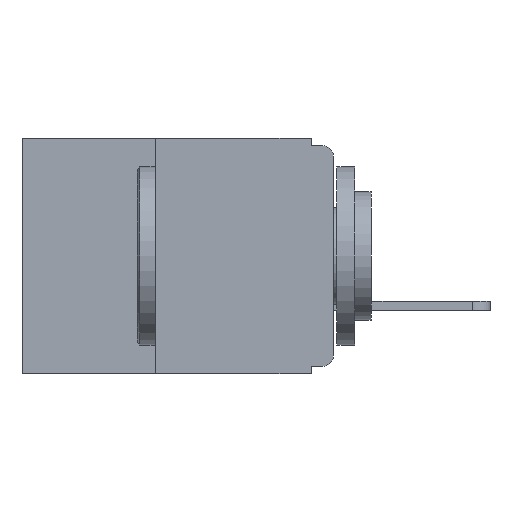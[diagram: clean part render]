
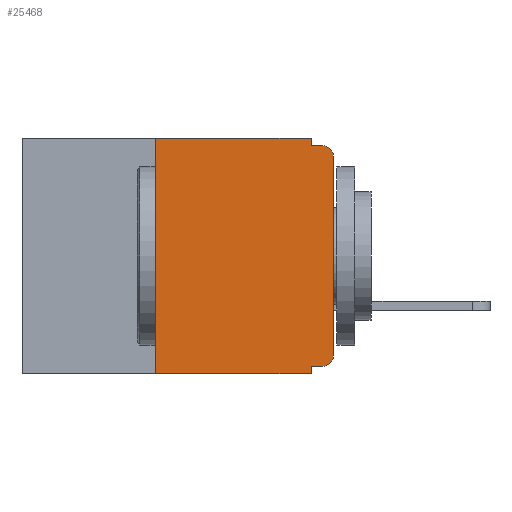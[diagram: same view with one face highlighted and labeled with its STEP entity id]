
A CAD part, left-side view. The second image highlights one B-rep face of the part: STEP entity #25468.
In plain terms, the highlighted planar face has unit normal (-1, 0, 0).
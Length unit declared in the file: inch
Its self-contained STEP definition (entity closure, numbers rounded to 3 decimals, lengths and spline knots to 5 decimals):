
#475 = CIRCLE ( 'NONE', #19467, 0.015 ) ;
#1059 = VERTEX_POINT ( 'NONE', #14954 ) ;
#1251 = DIRECTION ( 'NONE',  ( -1., 0., 0. ) ) ;
#1828 = LINE ( 'NONE', #4711, #18240 ) ;
#1950 = CARTESIAN_POINT ( 'NONE',  ( 0., 0.015, -0.32 ) ) ;
#2035 = AXIS2_PLACEMENT_3D ( 'NONE', #14182, #1251, #16287 ) ;
#2042 = CARTESIAN_POINT ( 'NONE',  ( 0., 0.437, 0. ) ) ;
#2110 = CARTESIAN_POINT ( 'NONE',  ( 0., 0., -0.01 ) ) ;
#2238 = CARTESIAN_POINT ( 'NONE',  ( 0., 0., 0. ) ) ;
#2360 = EDGE_CURVE ( 'NONE', #19780, #21510, #12543, .T. ) ;
#2605 = ORIENTED_EDGE ( 'NONE', *, *, #16018, .F. ) ;
#2923 = ORIENTED_EDGE ( 'NONE', *, *, #24044, .T. ) ;
#3243 = DIRECTION ( 'NONE',  ( -1., 0., 0. ) ) ;
#3440 = DIRECTION ( 'NONE',  ( 0., 0., 1. ) ) ;
#3784 = VECTOR ( 'NONE', #17156, 39.37008 ) ;
#4205 = DIRECTION ( 'NONE',  ( 1., 0., 0. ) ) ;
#4260 = DIRECTION ( 'NONE',  ( 0., -1., 0. ) ) ;
#4711 = CARTESIAN_POINT ( 'NONE',  ( 0., 0.437, -0.33 ) ) ;
#4857 = EDGE_LOOP ( 'NONE', ( #5251, #7624, #13266, #19024, #24674, #21934, #14259, #9284, #2605, #2923 ) ) ;
#5251 = ORIENTED_EDGE ( 'NONE', *, *, #25981, .T. ) ;
#5767 = LINE ( 'NONE', #27097, #15867 ) ;
#7027 = EDGE_CURVE ( 'NONE', #23904, #21510, #1828, .T. ) ;
#7468 = VECTOR ( 'NONE', #4260, 39.37008 ) ;
#7624 = ORIENTED_EDGE ( 'NONE', *, *, #8584, .T. ) ;
#7727 = VERTEX_POINT ( 'NONE', #25893 ) ;
#7881 = FACE_OUTER_BOUND ( 'NONE', #4857, .T. ) ;
#8262 = DIRECTION ( 'NONE',  ( 0., 1., 0. ) ) ;
#8273 = AXIS2_PLACEMENT_3D ( 'NONE', #2042, #4205, #19163 ) ;
#8584 = EDGE_CURVE ( 'NONE', #26038, #15516, #19142, .T. ) ;
#8741 = CARTESIAN_POINT ( 'NONE',  ( 0., 0.015, -0.01 ) ) ;
#9007 = DIRECTION ( 'NONE',  ( 0., -1., 0. ) ) ;
#9284 = ORIENTED_EDGE ( 'NONE', *, *, #2360, .F. ) ;
#9533 = VECTOR ( 'NONE', #8262, 39.37008 ) ;
#10306 = EDGE_CURVE ( 'NONE', #23904, #7727, #20723, .T. ) ;
#11213 = CARTESIAN_POINT ( 'NONE',  ( 0., 0.437, 0. ) ) ;
#11404 = CARTESIAN_POINT ( 'NONE',  ( 0., 0.25, -0.33 ) ) ;
#12468 = DIRECTION ( 'NONE',  ( 0., 0., -1. ) ) ;
#12543 = LINE ( 'NONE', #26912, #17462 ) ;
#13180 = CARTESIAN_POINT ( 'NONE',  ( 0., 0., -0.025 ) ) ;
#13212 = CARTESIAN_POINT ( 'NONE',  ( 0., 0.031, 0. ) ) ;
#13266 = ORIENTED_EDGE ( 'NONE', *, *, #16134, .F. ) ;
#14182 = CARTESIAN_POINT ( 'NONE',  ( 0., 0.015, -0.025 ) ) ;
#14259 = ORIENTED_EDGE ( 'NONE', *, *, #7027, .T. ) ;
#14548 = LINE ( 'NONE', #2110, #7468 ) ;
#14654 = CARTESIAN_POINT ( 'NONE',  ( 0., 0., -0.32 ) ) ;
#14953 = PLANE ( 'NONE',  #8273 ) ;
#14954 = CARTESIAN_POINT ( 'NONE',  ( 0., 0., -0.305 ) ) ;
#15505 = VECTOR ( 'NONE', #9007, 39.37008 ) ;
#15516 = VERTEX_POINT ( 'NONE', #8741 ) ;
#15772 = CARTESIAN_POINT ( 'NONE',  ( 0., 0.031, -0.32 ) ) ;
#15867 = VECTOR ( 'NONE', #12468, 39.37008 ) ;
#16018 = EDGE_CURVE ( 'NONE', #25443, #19780, #26955, .T. ) ;
#16100 = CARTESIAN_POINT ( 'NONE',  ( 0., 0.015, -0.305 ) ) ;
#16134 = EDGE_CURVE ( 'NONE', #24852, #15516, #14548, .T. ) ;
#16286 = CARTESIAN_POINT ( 'NONE',  ( 0., 0.25, -0.33 ) ) ;
#16287 = DIRECTION ( 'NONE',  ( 0., 0., -1. ) ) ;
#16823 = DIRECTION ( 'NONE',  ( 0., 0., -1. ) ) ;
#17156 = DIRECTION ( 'NONE',  ( 0., 0., 1. ) ) ;
#17462 = VECTOR ( 'NONE', #16823, 39.37008 ) ;
#17708 = EDGE_CURVE ( 'NONE', #21736, #24852, #5767, .T. ) ;
#18219 = DIRECTION ( 'NONE',  ( 0., 0., -1. ) ) ;
#18240 = VECTOR ( 'NONE', #21739, 39.37008 ) ;
#19024 = ORIENTED_EDGE ( 'NONE', *, *, #17708, .F. ) ;
#19142 = CIRCLE ( 'NONE', #2035, 0.015 ) ;
#19163 = DIRECTION ( 'NONE',  ( 0., 0., -1. ) ) ;
#19467 = AXIS2_PLACEMENT_3D ( 'NONE', #16100, #3243, #18219 ) ;
#19780 = VERTEX_POINT ( 'NONE', #15772 ) ;
#20723 = LINE ( 'NONE', #16286, #24654 ) ;
#21510 = VERTEX_POINT ( 'NONE', #24964 ) ;
#21696 = LINE ( 'NONE', #11213, #15505 ) ;
#21736 = VERTEX_POINT ( 'NONE', #13212 ) ;
#21739 = DIRECTION ( 'NONE',  ( 0., -1., 0. ) ) ;
#21934 = ORIENTED_EDGE ( 'NONE', *, *, #10306, .F. ) ;
#23904 = VERTEX_POINT ( 'NONE', #11404 ) ;
#24044 = EDGE_CURVE ( 'NONE', #25443, #1059, #475, .T. ) ;
#24654 = VECTOR ( 'NONE', #3440, 39.37008 ) ;
#24674 = ORIENTED_EDGE ( 'NONE', *, *, #26603, .F. ) ;
#24852 = VERTEX_POINT ( 'NONE', #24937 ) ;
#24937 = CARTESIAN_POINT ( 'NONE',  ( 0., 0.031, -0.01 ) ) ;
#24964 = CARTESIAN_POINT ( 'NONE',  ( 0., 0.031, -0.33 ) ) ;
#25443 = VERTEX_POINT ( 'NONE', #1950 ) ;
#25468 = ADVANCED_FACE ( 'NONE', ( #7881 ), #14953, .F. ) ;
#25655 = LINE ( 'NONE', #2238, #3784 ) ;
#25893 = CARTESIAN_POINT ( 'NONE',  ( 0., 0.25, 0. ) ) ;
#25981 = EDGE_CURVE ( 'NONE', #1059, #26038, #25655, .T. ) ;
#26038 = VERTEX_POINT ( 'NONE', #13180 ) ;
#26603 = EDGE_CURVE ( 'NONE', #7727, #21736, #21696, .T. ) ;
#26912 = CARTESIAN_POINT ( 'NONE',  ( 0., 0.031, -0.33 ) ) ;
#26955 = LINE ( 'NONE', #14654, #9533 ) ;
#27097 = CARTESIAN_POINT ( 'NONE',  ( 0., 0.031, 0. ) ) ;
